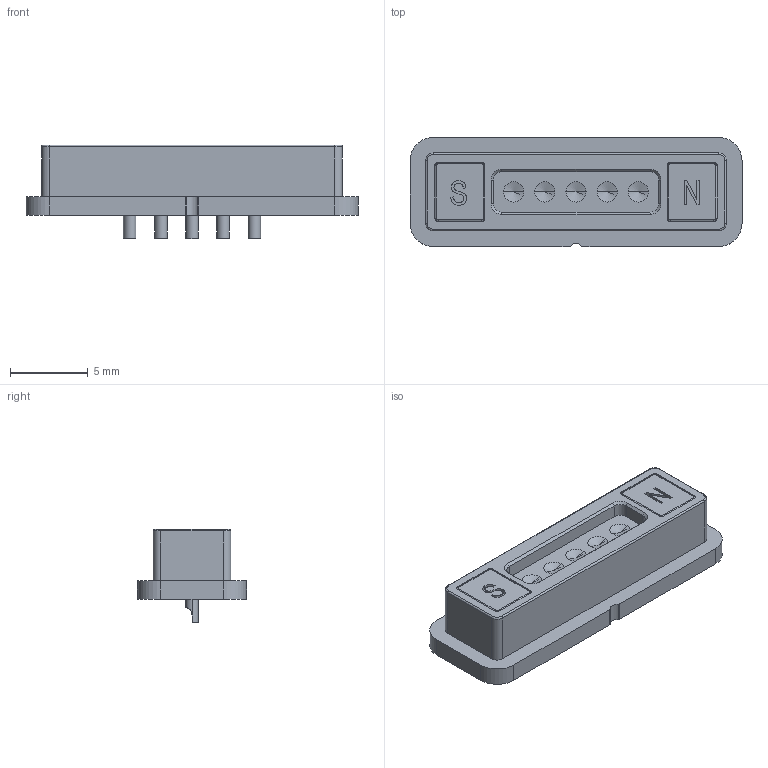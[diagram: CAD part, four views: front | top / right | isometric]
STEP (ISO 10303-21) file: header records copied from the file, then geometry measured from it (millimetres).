
FILE_DESCRIPTION (( 'STEP AP203' ), '1' );
FILE_NAME ('686-J0521450110.STEP', '2023-02-14T12:19:03', ( 'Magnum' ), ( '' ), 'SwSTEP 2.0', 'SolidWorks 2020', '' );
FILE_SCHEMA (( 'CONFIG_CONTROL_DESIGN' ));
Length unit declared in the file: millimetre
Products named in the file (1): 686-J0521450110
Bounding box: 21.3 x 7 x 6 mm (x, y, z)
Volume: 428.3 mm3; surface area: 684.3 mm2
Topology: 6 solids, 8 shells, 246 faces, 590 edges, 350 vertices
Faces by surface type: plane 95, cylinder 86, cone 31, bspline 20, torus 14
Entity records: 8235 total; most frequent: CARTESIAN_POINT 2587, DIRECTION 1173, ORIENTED_EDGE 1130, EDGE_CURVE 565, AXIS2_PLACEMENT_3D 419, VERTEX_POINT 350, LINE 335, VECTOR 335
